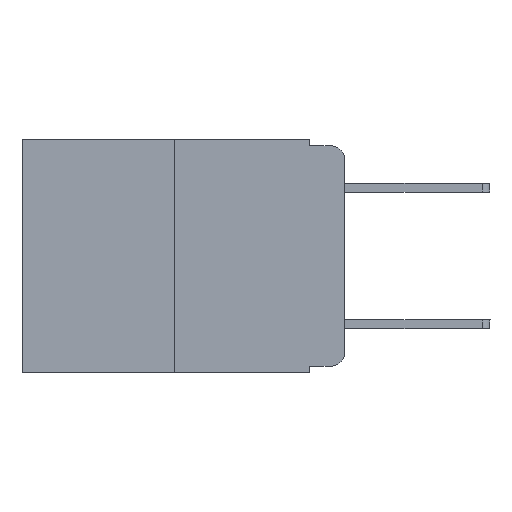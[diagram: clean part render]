
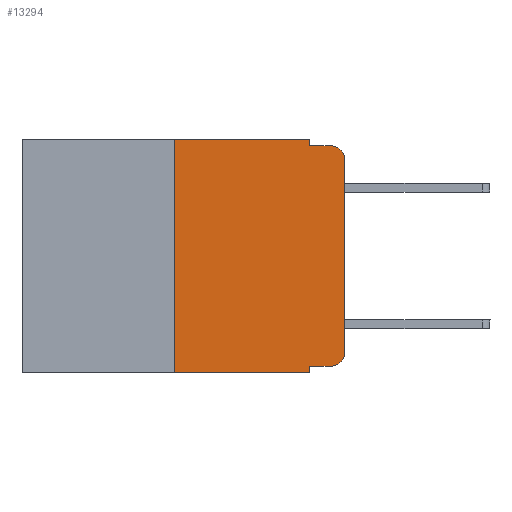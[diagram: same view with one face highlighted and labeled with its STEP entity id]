
A CAD part, left-side view. The second image highlights one B-rep face of the part: STEP entity #13294.
In plain terms, the highlighted planar face has unit normal (-1, 0, 0).
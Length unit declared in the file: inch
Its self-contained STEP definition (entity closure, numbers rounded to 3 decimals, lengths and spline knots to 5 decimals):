
#241 = VECTOR ( 'NONE', #5607, 39.37008 ) ;
#639 = CARTESIAN_POINT ( 'NONE',  ( 0., 0.051, -0.333 ) ) ;
#1311 = CIRCLE ( 'NONE', #6987, 0.02 ) ;
#1885 = CARTESIAN_POINT ( 'NONE',  ( 0., 0.051, -0.01 ) ) ;
#1924 = EDGE_CURVE ( 'NONE', #7678, #10640, #7724, .T. ) ;
#2443 = EDGE_CURVE ( 'NONE', #17209, #16545, #8753, .T. ) ;
#2551 = LINE ( 'NONE', #8399, #6497 ) ;
#2571 = LINE ( 'NONE', #19269, #10405 ) ;
#2592 = VECTOR ( 'NONE', #3309, 39.37008 ) ;
#2711 = ORIENTED_EDGE ( 'NONE', *, *, #11679, .F. ) ;
#2768 = DIRECTION ( 'NONE',  ( 1., 0., 0. ) ) ;
#2863 = ORIENTED_EDGE ( 'NONE', *, *, #8172, .F. ) ;
#3228 = CARTESIAN_POINT ( 'NONE',  ( 0., 0.02, -0.03 ) ) ;
#3309 = DIRECTION ( 'NONE',  ( 0., -1., 0. ) ) ;
#3496 = AXIS2_PLACEMENT_3D ( 'NONE', #12646, #2768, #14467 ) ;
#3614 = LINE ( 'NONE', #21524, #2592 ) ;
#3959 = CARTESIAN_POINT ( 'NONE',  ( 0., 0.25, 0. ) ) ;
#4240 = DIRECTION ( 'NONE',  ( 0., -1., 0. ) ) ;
#4329 = CARTESIAN_POINT ( 'NONE',  ( 0., 0.051, 0. ) ) ;
#4650 = CIRCLE ( 'NONE', #8797, 0.02 ) ;
#4802 = DIRECTION ( 'NONE',  ( 0., 0., -1. ) ) ;
#5089 = DIRECTION ( 'NONE',  ( 0., -1., 0. ) ) ;
#5132 = DIRECTION ( 'NONE',  ( 0., 0., -1. ) ) ;
#5607 = DIRECTION ( 'NONE',  ( 0., 0., 1. ) ) ;
#5800 = CARTESIAN_POINT ( 'NONE',  ( 0., 0., 0. ) ) ;
#6118 = DIRECTION ( 'NONE',  ( -1., 0., 0. ) ) ;
#6294 = LINE ( 'NONE', #3959, #241 ) ;
#6497 = VECTOR ( 'NONE', #5089, 39.37008 ) ;
#6705 = DIRECTION ( 'NONE',  ( -1., 0., 0. ) ) ;
#6987 = AXIS2_PLACEMENT_3D ( 'NONE', #16123, #6118, #19501 ) ;
#7064 = EDGE_CURVE ( 'NONE', #15802, #9900, #2551, .T. ) ;
#7231 = CARTESIAN_POINT ( 'NONE',  ( 0., 0., -0.03 ) ) ;
#7678 = VERTEX_POINT ( 'NONE', #639 ) ;
#7724 = LINE ( 'NONE', #14430, #16326 ) ;
#7744 = ORIENTED_EDGE ( 'NONE', *, *, #18758, .T. ) ;
#7747 = CARTESIAN_POINT ( 'NONE',  ( 0., 0.02, -0.01 ) ) ;
#8172 = EDGE_CURVE ( 'NONE', #11861, #15802, #10363, .T. ) ;
#8399 = CARTESIAN_POINT ( 'NONE',  ( 0., 0.051, -0.01 ) ) ;
#8662 = DIRECTION ( 'NONE',  ( 0., 0., -1. ) ) ;
#8753 = LINE ( 'NONE', #5800, #16575 ) ;
#8797 = AXIS2_PLACEMENT_3D ( 'NONE', #3228, #6705, #8662 ) ;
#9632 = FACE_OUTER_BOUND ( 'NONE', #18018, .T. ) ;
#9900 = VERTEX_POINT ( 'NONE', #7747 ) ;
#10121 = ORIENTED_EDGE ( 'NONE', *, *, #7064, .F. ) ;
#10159 = CARTESIAN_POINT ( 'NONE',  ( 0., 0.25, -0.343 ) ) ;
#10363 = LINE ( 'NONE', #13295, #21321 ) ;
#10405 = VECTOR ( 'NONE', #17741, 39.37008 ) ;
#10640 = VERTEX_POINT ( 'NONE', #14357 ) ;
#10791 = EDGE_CURVE ( 'NONE', #7678, #18716, #17846, .T. ) ;
#11679 = EDGE_CURVE ( 'NONE', #18355, #14704, #6294, .T. ) ;
#11721 = CARTESIAN_POINT ( 'NONE',  ( 0., 0.051, 0. ) ) ;
#11861 = VERTEX_POINT ( 'NONE', #4329 ) ;
#12309 = ORIENTED_EDGE ( 'NONE', *, *, #2443, .T. ) ;
#12646 = CARTESIAN_POINT ( 'NONE',  ( 0., 0.473, 0. ) ) ;
#12818 = ORIENTED_EDGE ( 'NONE', *, *, #18136, .T. ) ;
#13294 = ADVANCED_FACE ( 'NONE', ( #9632 ), #19451, .F. ) ;
#13295 = CARTESIAN_POINT ( 'NONE',  ( 0., 0.051, 0. ) ) ;
#13418 = ORIENTED_EDGE ( 'NONE', *, *, #10791, .F. ) ;
#14357 = CARTESIAN_POINT ( 'NONE',  ( 0., 0.02, -0.333 ) ) ;
#14405 = ORIENTED_EDGE ( 'NONE', *, *, #1924, .T. ) ;
#14430 = CARTESIAN_POINT ( 'NONE',  ( 0., 0.051, -0.333 ) ) ;
#14467 = DIRECTION ( 'NONE',  ( 0., 0., -1. ) ) ;
#14704 = VERTEX_POINT ( 'NONE', #18528 ) ;
#15802 = VERTEX_POINT ( 'NONE', #1885 ) ;
#16123 = CARTESIAN_POINT ( 'NONE',  ( 0., 0.02, -0.313 ) ) ;
#16239 = CARTESIAN_POINT ( 'NONE',  ( 0., 0.051, -0.343 ) ) ;
#16326 = VECTOR ( 'NONE', #4240, 39.37008 ) ;
#16391 = ORIENTED_EDGE ( 'NONE', *, *, #21179, .F. ) ;
#16545 = VERTEX_POINT ( 'NONE', #7231 ) ;
#16575 = VECTOR ( 'NONE', #17507, 39.37008 ) ;
#17209 = VERTEX_POINT ( 'NONE', #20596 ) ;
#17507 = DIRECTION ( 'NONE',  ( 0., 0., 1. ) ) ;
#17741 = DIRECTION ( 'NONE',  ( 0., -1., 0. ) ) ;
#17846 = LINE ( 'NONE', #11721, #18108 ) ;
#18018 = EDGE_LOOP ( 'NONE', ( #12309, #7744, #10121, #2863, #16391, #2711, #12818, #13418, #14405, #19030 ) ) ;
#18062 = EDGE_CURVE ( 'NONE', #10640, #17209, #1311, .T. ) ;
#18108 = VECTOR ( 'NONE', #5132, 39.37008 ) ;
#18136 = EDGE_CURVE ( 'NONE', #18355, #18716, #3614, .T. ) ;
#18355 = VERTEX_POINT ( 'NONE', #10159 ) ;
#18528 = CARTESIAN_POINT ( 'NONE',  ( 0., 0.25, 0. ) ) ;
#18716 = VERTEX_POINT ( 'NONE', #16239 ) ;
#18758 = EDGE_CURVE ( 'NONE', #16545, #9900, #4650, .T. ) ;
#19030 = ORIENTED_EDGE ( 'NONE', *, *, #18062, .T. ) ;
#19269 = CARTESIAN_POINT ( 'NONE',  ( 0., 0.473, 0. ) ) ;
#19451 = PLANE ( 'NONE',  #3496 ) ;
#19501 = DIRECTION ( 'NONE',  ( 0., 0., -1. ) ) ;
#20596 = CARTESIAN_POINT ( 'NONE',  ( 0., 0., -0.313 ) ) ;
#21179 = EDGE_CURVE ( 'NONE', #14704, #11861, #2571, .T. ) ;
#21321 = VECTOR ( 'NONE', #4802, 39.37008 ) ;
#21524 = CARTESIAN_POINT ( 'NONE',  ( 0., 0.473, -0.343 ) ) ;
